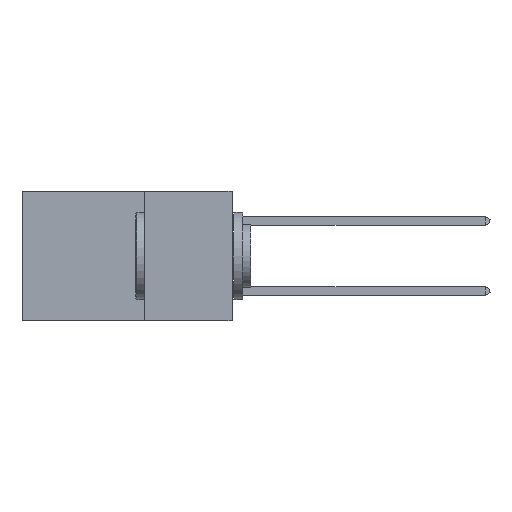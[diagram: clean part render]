
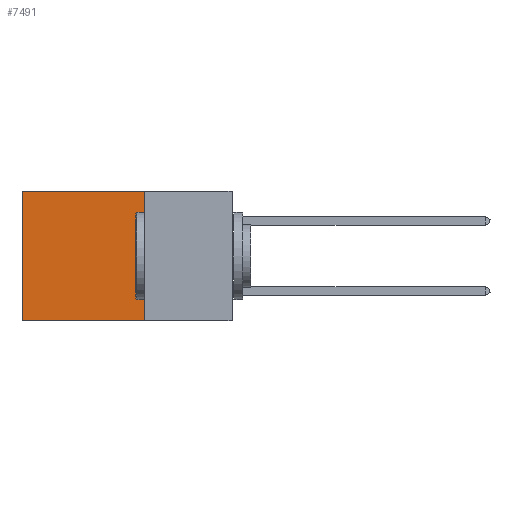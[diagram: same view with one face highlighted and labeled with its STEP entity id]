
A CAD part, left-side view. The second image highlights one B-rep face of the part: STEP entity #7491.
In plain terms, the highlighted planar face has unit normal (-1, 0, 0).
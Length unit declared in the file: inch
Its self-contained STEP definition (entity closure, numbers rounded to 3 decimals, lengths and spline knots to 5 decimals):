
#854 = EDGE_LOOP ( 'NONE', ( #28301, #29295, #32283, #17931 ) ) ;
#4144 = LINE ( 'NONE', #13101, #37754 ) ;
#4982 = VECTOR ( 'NONE', #35980, 39.37008 ) ;
#5182 = FACE_OUTER_BOUND ( 'NONE', #854, .T. ) ;
#6370 = LINE ( 'NONE', #24210, #4982 ) ;
#6922 = VECTOR ( 'NONE', #27350, 39.37008 ) ;
#7491 = ADVANCED_FACE ( 'NONE', ( #5182 ), #16235, .F. ) ;
#10682 = VERTEX_POINT ( 'NONE', #15889 ) ;
#13101 = CARTESIAN_POINT ( 'NONE',  ( 0.2875, 0.25, -0.37 ) ) ;
#13381 = EDGE_CURVE ( 'NONE', #10682, #15608, #13526, .T. ) ;
#13526 = LINE ( 'NONE', #37128, #21476 ) ;
#15608 = VERTEX_POINT ( 'NONE', #24640 ) ;
#15889 = CARTESIAN_POINT ( 'NONE',  ( 0.2875, 0.25, 0. ) ) ;
#16235 = PLANE ( 'NONE',  #35785 ) ;
#17931 = ORIENTED_EDGE ( 'NONE', *, *, #13381, .T. ) ;
#18847 = DIRECTION ( 'NONE',  ( 0., 1., 0. ) ) ;
#19264 = CARTESIAN_POINT ( 'NONE',  ( 0.2875, 0.6, -0.37 ) ) ;
#19374 = CARTESIAN_POINT ( 'NONE',  ( 0.2875, 0.25, 0. ) ) ;
#21446 = EDGE_CURVE ( 'NONE', #23167, #24367, #4144, .T. ) ;
#21476 = VECTOR ( 'NONE', #18847, 39.37008 ) ;
#21836 = DIRECTION ( 'NONE',  ( 0., 1., 0. ) ) ;
#21863 = LINE ( 'NONE', #27216, #6922 ) ;
#22566 = EDGE_CURVE ( 'NONE', #15608, #24367, #6370, .T. ) ;
#22604 = CARTESIAN_POINT ( 'NONE',  ( 0.2875, 0.25, -0.37 ) ) ;
#23167 = VERTEX_POINT ( 'NONE', #22604 ) ;
#24210 = CARTESIAN_POINT ( 'NONE',  ( 0.2875, 0.6, 0. ) ) ;
#24367 = VERTEX_POINT ( 'NONE', #19264 ) ;
#24640 = CARTESIAN_POINT ( 'NONE',  ( 0.2875, 0.6, 0. ) ) ;
#25525 = DIRECTION ( 'NONE',  ( 1., 0., 0. ) ) ;
#27216 = CARTESIAN_POINT ( 'NONE',  ( 0.2875, 0.25, 0. ) ) ;
#27350 = DIRECTION ( 'NONE',  ( 0., 0., -1. ) ) ;
#28301 = ORIENTED_EDGE ( 'NONE', *, *, #22566, .T. ) ;
#28390 = DIRECTION ( 'NONE',  ( 0., 0., -1. ) ) ;
#28815 = EDGE_CURVE ( 'NONE', #10682, #23167, #21863, .T. ) ;
#29295 = ORIENTED_EDGE ( 'NONE', *, *, #21446, .F. ) ;
#32283 = ORIENTED_EDGE ( 'NONE', *, *, #28815, .F. ) ;
#35785 = AXIS2_PLACEMENT_3D ( 'NONE', #19374, #25525, #28390 ) ;
#35980 = DIRECTION ( 'NONE',  ( 0., 0., -1. ) ) ;
#37128 = CARTESIAN_POINT ( 'NONE',  ( 0.2875, 0.25, 0. ) ) ;
#37754 = VECTOR ( 'NONE', #21836, 39.37008 ) ;
